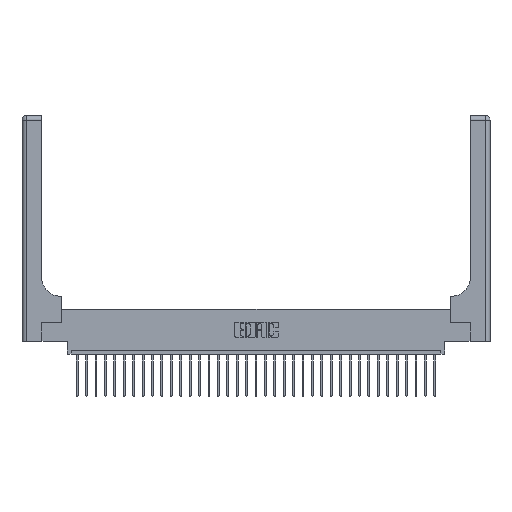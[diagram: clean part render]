
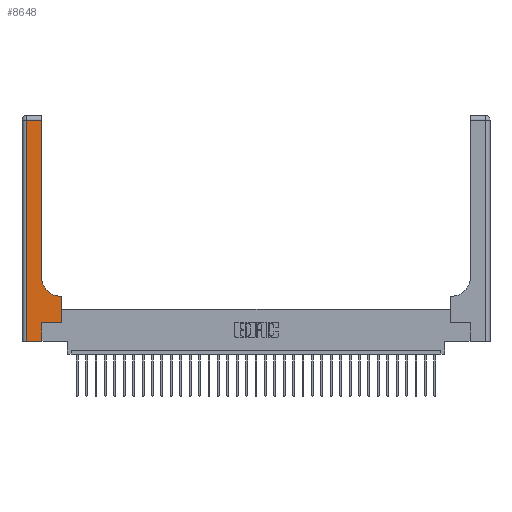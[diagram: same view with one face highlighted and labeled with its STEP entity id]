
A CAD part, top view. The second image highlights one B-rep face of the part: STEP entity #8648.
In plain terms, the highlighted planar face has unit normal (0, 0, 1).
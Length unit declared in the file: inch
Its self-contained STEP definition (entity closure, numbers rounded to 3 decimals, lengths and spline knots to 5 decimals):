
#78 = EDGE_CURVE ( 'NONE', #8455, #17413, #22065, .T. ) ;
#350 = VERTEX_POINT ( 'NONE', #1808 ) ;
#352 = AXIS2_PLACEMENT_3D ( 'NONE', #18751, #23348, #27969 ) ;
#547 = VERTEX_POINT ( 'NONE', #9169 ) ;
#1397 = VERTEX_POINT ( 'NONE', #13023 ) ;
#1808 = CARTESIAN_POINT ( 'NONE',  ( 0.26, 2.94, 0.37 ) ) ;
#2041 = CARTESIAN_POINT ( 'NONE',  ( 0.51, 0.6, 0.37 ) ) ;
#2298 = ORIENTED_EDGE ( 'NONE', *, *, #7274, .T. ) ;
#2694 = LINE ( 'NONE', #4304, #8897 ) ;
#3065 = LINE ( 'NONE', #13565, #12167 ) ;
#3277 = VECTOR ( 'NONE', #25748, 39.37008 ) ;
#3436 = DIRECTION ( 'NONE',  ( 0., 0., -1. ) ) ;
#3945 = EDGE_CURVE ( 'NONE', #350, #1397, #2694, .T. ) ;
#3974 = ORIENTED_EDGE ( 'NONE', *, *, #13501, .T. ) ;
#4304 = CARTESIAN_POINT ( 'NONE',  ( 0., 2.94, 0.37 ) ) ;
#4327 = VERTEX_POINT ( 'NONE', #2041 ) ;
#4497 = CARTESIAN_POINT ( 'NONE',  ( 0.528, 0.25, 0.37 ) ) ;
#5464 = DIRECTION ( 'NONE',  ( 1., 0., 0. ) ) ;
#7274 = EDGE_CURVE ( 'NONE', #547, #350, #17932, .T. ) ;
#7827 = ORIENTED_EDGE ( 'NONE', *, *, #11043, .T. ) ;
#8455 = VERTEX_POINT ( 'NONE', #4497 ) ;
#8504 = EDGE_CURVE ( 'NONE', #1397, #15746, #12448, .T. ) ;
#8648 = ADVANCED_FACE ( 'NONE', ( #25377 ), #27289, .F. ) ;
#8897 = VECTOR ( 'NONE', #8992, 39.37008 ) ;
#8961 = VECTOR ( 'NONE', #9554, 39.37008 ) ;
#8992 = DIRECTION ( 'NONE',  ( -1., 0., 0. ) ) ;
#9169 = CARTESIAN_POINT ( 'NONE',  ( 0.26, 0.85, 0.37 ) ) ;
#9554 = DIRECTION ( 'NONE',  ( -1., 0., 0. ) ) ;
#9563 = CARTESIAN_POINT ( 'NONE',  ( 0.265, 0., 0.37 ) ) ;
#9644 = EDGE_CURVE ( 'NONE', #19012, #10897, #21745, .T. ) ;
#10015 = VECTOR ( 'NONE', #5464, 39.37008 ) ;
#10448 = CARTESIAN_POINT ( 'NONE',  ( 0.26, 3., 0.37 ) ) ;
#10639 = VECTOR ( 'NONE', #21088, 39.37008 ) ;
#10897 = VERTEX_POINT ( 'NONE', #25769 ) ;
#11043 = EDGE_CURVE ( 'NONE', #4327, #547, #22354, .T. ) ;
#11475 = ORIENTED_EDGE ( 'NONE', *, *, #21750, .T. ) ;
#11932 = CARTESIAN_POINT ( 'NONE',  ( 0.06, 3., 0.37 ) ) ;
#12167 = VECTOR ( 'NONE', #29635, 39.37008 ) ;
#12448 = LINE ( 'NONE', #11932, #10639 ) ;
#13023 = CARTESIAN_POINT ( 'NONE',  ( 0.06, 2.94, 0.37 ) ) ;
#13501 = EDGE_CURVE ( 'NONE', #10897, #8455, #3065, .T. ) ;
#13565 = CARTESIAN_POINT ( 'NONE',  ( 0.265, 0.25, 0.37 ) ) ;
#14228 = CARTESIAN_POINT ( 'NONE',  ( 0.26, 0.6, 0.37 ) ) ;
#14946 = CARTESIAN_POINT ( 'NONE',  ( 0.51, 0.85, 0.37 ) ) ;
#14985 = AXIS2_PLACEMENT_3D ( 'NONE', #14946, #3436, #19661 ) ;
#15108 = DIRECTION ( 'NONE',  ( 0., 1., 0. ) ) ;
#15132 = LINE ( 'NONE', #14228, #8961 ) ;
#15746 = VERTEX_POINT ( 'NONE', #19818 ) ;
#16003 = VECTOR ( 'NONE', #22089, 39.37008 ) ;
#17250 = ORIENTED_EDGE ( 'NONE', *, *, #78, .T. ) ;
#17413 = VERTEX_POINT ( 'NONE', #28545 ) ;
#17932 = LINE ( 'NONE', #10448, #20798 ) ;
#18720 = LINE ( 'NONE', #21961, #10015 ) ;
#18751 = CARTESIAN_POINT ( 'NONE',  ( 0., 3., 0.37 ) ) ;
#19012 = VERTEX_POINT ( 'NONE', #29315 ) ;
#19620 = ORIENTED_EDGE ( 'NONE', *, *, #8504, .T. ) ;
#19661 = DIRECTION ( 'NONE',  ( 1., 0., 0. ) ) ;
#19809 = CARTESIAN_POINT ( 'NONE',  ( 0.528, 0.25, 0.37 ) ) ;
#19818 = CARTESIAN_POINT ( 'NONE',  ( 0.06, 0., 0.37 ) ) ;
#20798 = VECTOR ( 'NONE', #15108, 39.37008 ) ;
#21088 = DIRECTION ( 'NONE',  ( 0., -1., 0. ) ) ;
#21745 = LINE ( 'NONE', #9563, #3277 ) ;
#21750 = EDGE_CURVE ( 'NONE', #17413, #4327, #15132, .T. ) ;
#21961 = CARTESIAN_POINT ( 'NONE',  ( 0., 0., 0.37 ) ) ;
#22065 = LINE ( 'NONE', #19809, #16003 ) ;
#22089 = DIRECTION ( 'NONE',  ( 0., 1., 0. ) ) ;
#22354 = CIRCLE ( 'NONE', #14985, 0.25 ) ;
#22606 = ORIENTED_EDGE ( 'NONE', *, *, #24075, .T. ) ;
#23348 = DIRECTION ( 'NONE',  ( 0., 0., -1. ) ) ;
#23780 = EDGE_LOOP ( 'NONE', ( #2298, #29166, #19620, #22606, #26209, #3974, #17250, #11475, #7827 ) ) ;
#24075 = EDGE_CURVE ( 'NONE', #15746, #19012, #18720, .T. ) ;
#25377 = FACE_OUTER_BOUND ( 'NONE', #23780, .T. ) ;
#25748 = DIRECTION ( 'NONE',  ( 0., 1., 0. ) ) ;
#25769 = CARTESIAN_POINT ( 'NONE',  ( 0.265, 0.25, 0.37 ) ) ;
#26209 = ORIENTED_EDGE ( 'NONE', *, *, #9644, .T. ) ;
#27289 = PLANE ( 'NONE',  #352 ) ;
#27969 = DIRECTION ( 'NONE',  ( -1., 0., 0. ) ) ;
#28545 = CARTESIAN_POINT ( 'NONE',  ( 0.528, 0.6, 0.37 ) ) ;
#29166 = ORIENTED_EDGE ( 'NONE', *, *, #3945, .T. ) ;
#29315 = CARTESIAN_POINT ( 'NONE',  ( 0.265, 0., 0.37 ) ) ;
#29635 = DIRECTION ( 'NONE',  ( 1., 0., 0. ) ) ;
